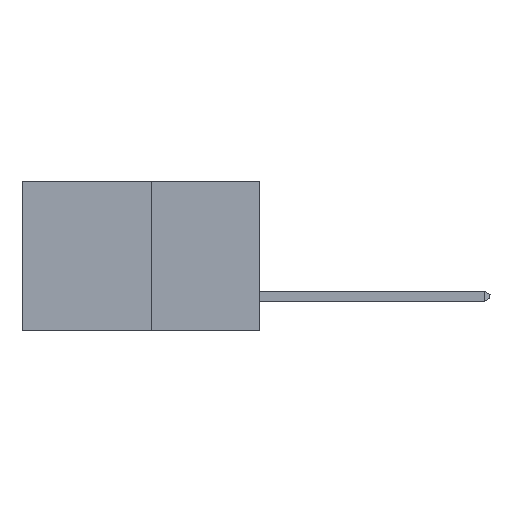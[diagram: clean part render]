
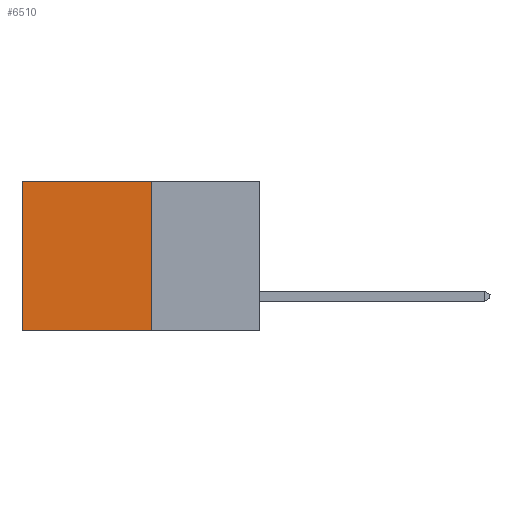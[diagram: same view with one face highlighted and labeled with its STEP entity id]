
A CAD part, left-side view. The second image highlights one B-rep face of the part: STEP entity #6510.
In plain terms, the highlighted planar face has unit normal (-1, 0, 0).
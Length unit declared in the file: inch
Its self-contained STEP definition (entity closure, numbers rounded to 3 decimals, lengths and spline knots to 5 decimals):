
#689 = ORIENTED_EDGE ( 'NONE', *, *, #4839, .T. ) ;
#2127 = VERTEX_POINT ( 'NONE', #29140 ) ;
#3270 = CARTESIAN_POINT ( 'NONE',  ( 0.277, 0.27, 0. ) ) ;
#4558 = VERTEX_POINT ( 'NONE', #3270 ) ;
#4839 = EDGE_CURVE ( 'NONE', #4558, #2127, #15217, .T. ) ;
#5377 = PLANE ( 'NONE',  #14757 ) ;
#5524 = DIRECTION ( 'NONE',  ( 0., 0., -1. ) ) ;
#5800 = ORIENTED_EDGE ( 'NONE', *, *, #21999, .F. ) ;
#6510 = ADVANCED_FACE ( 'NONE', ( #13365 ), #5377, .F. ) ;
#7880 = DIRECTION ( 'NONE',  ( 1., 0., 0. ) ) ;
#7896 = VECTOR ( 'NONE', #14232, 39.37008 ) ;
#9694 = VECTOR ( 'NONE', #17571, 39.37008 ) ;
#10471 = LINE ( 'NONE', #22403, #9694 ) ;
#10638 = VECTOR ( 'NONE', #5524, 39.37008 ) ;
#11272 = CARTESIAN_POINT ( 'NONE',  ( 0.277, 0.27, -0.37 ) ) ;
#12774 = CARTESIAN_POINT ( 'NONE',  ( 0.277, 0.27, -0.37 ) ) ;
#13365 = FACE_OUTER_BOUND ( 'NONE', #15416, .T. ) ;
#14232 = DIRECTION ( 'NONE',  ( 0., 1., 0. ) ) ;
#14757 = AXIS2_PLACEMENT_3D ( 'NONE', #12774, #7880, #24871 ) ;
#15217 = LINE ( 'NONE', #26229, #7896 ) ;
#15416 = EDGE_LOOP ( 'NONE', ( #28384, #16913, #5800, #689 ) ) ;
#16795 = VECTOR ( 'NONE', #18043, 39.37008 ) ;
#16913 = ORIENTED_EDGE ( 'NONE', *, *, #26039, .F. ) ;
#17571 = DIRECTION ( 'NONE',  ( 0., 1., 0. ) ) ;
#18043 = DIRECTION ( 'NONE',  ( 0., 0., -1. ) ) ;
#21999 = EDGE_CURVE ( 'NONE', #4558, #27165, #30595, .T. ) ;
#22204 = EDGE_CURVE ( 'NONE', #2127, #25201, #23145, .T. ) ;
#22403 = CARTESIAN_POINT ( 'NONE',  ( 0.277, 0.27, -0.37 ) ) ;
#22639 = CARTESIAN_POINT ( 'NONE',  ( 0.277, 0.27, -0.37 ) ) ;
#23145 = LINE ( 'NONE', #27540, #16795 ) ;
#23981 = CARTESIAN_POINT ( 'NONE',  ( 0.277, 0.59, -0.37 ) ) ;
#24871 = DIRECTION ( 'NONE',  ( 0., 0., -1. ) ) ;
#25201 = VERTEX_POINT ( 'NONE', #23981 ) ;
#26039 = EDGE_CURVE ( 'NONE', #27165, #25201, #10471, .T. ) ;
#26229 = CARTESIAN_POINT ( 'NONE',  ( 0.277, 0.27, 0. ) ) ;
#27165 = VERTEX_POINT ( 'NONE', #11272 ) ;
#27540 = CARTESIAN_POINT ( 'NONE',  ( 0.277, 0.59, -0.37 ) ) ;
#28384 = ORIENTED_EDGE ( 'NONE', *, *, #22204, .T. ) ;
#29140 = CARTESIAN_POINT ( 'NONE',  ( 0.277, 0.59, 0. ) ) ;
#30595 = LINE ( 'NONE', #22639, #10638 ) ;
